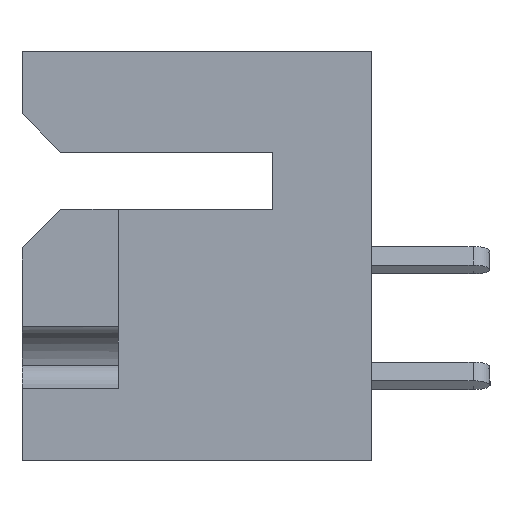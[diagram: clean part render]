
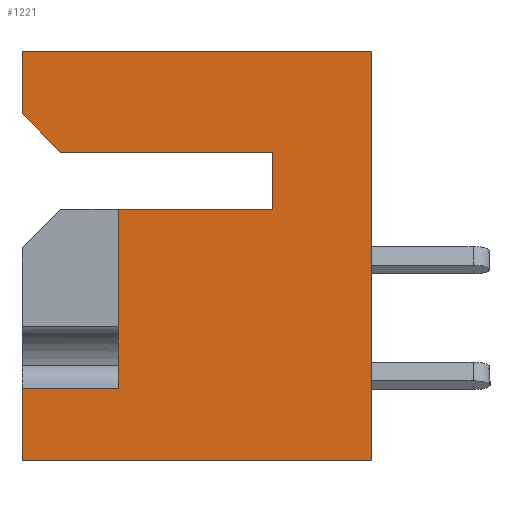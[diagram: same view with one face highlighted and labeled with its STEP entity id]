
A CAD part, left-side view. The second image highlights one B-rep face of the part: STEP entity #1221.
In plain terms, the highlighted planar face has unit normal (-1, 0, 0).
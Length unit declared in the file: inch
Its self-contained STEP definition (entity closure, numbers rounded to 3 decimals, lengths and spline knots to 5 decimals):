
#362 = DIRECTION ( 'NONE',  ( 0., 1., 0. ) ) ;
#945 = VECTOR ( 'NONE', #14442, 39.37008 ) ;
#1119 = ORIENTED_EDGE ( 'NONE', *, *, #4500, .T. ) ;
#1132 = EDGE_CURVE ( 'NONE', #11467, #28084, #12028, .T. ) ;
#1145 = CARTESIAN_POINT ( 'NONE',  ( 0., 0.453, -0.437 ) ) ;
#1221 = ADVANCED_FACE ( 'NONE', ( #16175 ), #7892, .F. ) ;
#1493 = LINE ( 'NONE', #23773, #14653 ) ;
#1674 = AXIS2_PLACEMENT_3D ( 'NONE', #18499, #18599, #3342 ) ;
#2130 = CARTESIAN_POINT ( 'NONE',  ( 0., 0., 0. ) ) ;
#2176 = VECTOR ( 'NONE', #12810, 39.37008 ) ;
#2653 = VECTOR ( 'NONE', #13168, 39.37008 ) ;
#2753 = DIRECTION ( 'NONE',  ( 0., 0., 1. ) ) ;
#3054 = CARTESIAN_POINT ( 'NONE',  ( 0., 0.328, -0.205 ) ) ;
#3342 = DIRECTION ( 'NONE',  ( 0., 0., -1. ) ) ;
#3590 = CARTESIAN_POINT ( 'NONE',  ( 0., 0.453, -0.531 ) ) ;
#3618 = DIRECTION ( 'NONE',  ( 0., 1., 0. ) ) ;
#3740 = EDGE_CURVE ( 'NONE', #21282, #23995, #8416, .T. ) ;
#3867 = LINE ( 'NONE', #22936, #25916 ) ;
#4013 = CARTESIAN_POINT ( 'NONE',  ( 0., 0.128, -0.131 ) ) ;
#4500 = EDGE_CURVE ( 'NONE', #8848, #18688, #3867, .T. ) ;
#4705 = CARTESIAN_POINT ( 'NONE',  ( 0., 0.128, -0.131 ) ) ;
#5362 = VECTOR ( 'NONE', #2753, 39.37008 ) ;
#6960 = EDGE_CURVE ( 'NONE', #21282, #28044, #8560, .T. ) ;
#7069 = CARTESIAN_POINT ( 'NONE',  ( 0., 0.328, -0.437 ) ) ;
#7250 = EDGE_CURVE ( 'NONE', #8031, #23120, #27135, .T. ) ;
#7589 = VECTOR ( 'NONE', #8153, 39.37008 ) ;
#7639 = EDGE_CURVE ( 'NONE', #23120, #28044, #24758, .T. ) ;
#7892 = PLANE ( 'NONE',  #1674 ) ;
#8031 = VERTEX_POINT ( 'NONE', #22704 ) ;
#8153 = DIRECTION ( 'NONE',  ( 0., 0., 1. ) ) ;
#8416 = LINE ( 'NONE', #19460, #2176 ) ;
#8560 = LINE ( 'NONE', #8652, #2653 ) ;
#8652 = CARTESIAN_POINT ( 'NONE',  ( 0., 0.403, -0.131 ) ) ;
#8705 = EDGE_CURVE ( 'NONE', #18688, #21297, #10562, .T. ) ;
#8848 = VERTEX_POINT ( 'NONE', #3590 ) ;
#9035 = VECTOR ( 'NONE', #362, 39.37008 ) ;
#9181 = CARTESIAN_POINT ( 'NONE',  ( 0., 0.328, -0.205 ) ) ;
#9204 = VERTEX_POINT ( 'NONE', #1145 ) ;
#9658 = EDGE_CURVE ( 'NONE', #8848, #9204, #23462, .T. ) ;
#10082 = VECTOR ( 'NONE', #25628, 39.37008 ) ;
#10555 = CARTESIAN_POINT ( 'NONE',  ( 0., 0.453, 0. ) ) ;
#10562 = LINE ( 'NONE', #13758, #5362 ) ;
#11389 = DIRECTION ( 'NONE',  ( 0., 0., 1. ) ) ;
#11467 = VERTEX_POINT ( 'NONE', #19345 ) ;
#12028 = LINE ( 'NONE', #3054, #945 ) ;
#12146 = LINE ( 'NONE', #19001, #10082 ) ;
#12249 = ORIENTED_EDGE ( 'NONE', *, *, #22726, .F. ) ;
#12333 = VECTOR ( 'NONE', #3618, 39.37008 ) ;
#12810 = DIRECTION ( 'NONE',  ( 0., 0., 1. ) ) ;
#12942 = CARTESIAN_POINT ( 'NONE',  ( 0., 0.403, -0.131 ) ) ;
#13168 = DIRECTION ( 'NONE',  ( 0., -0.707, -0.707 ) ) ;
#13758 = CARTESIAN_POINT ( 'NONE',  ( 0., 0., 0. ) ) ;
#13984 = DIRECTION ( 'NONE',  ( 0., -1., 0. ) ) ;
#14442 = DIRECTION ( 'NONE',  ( 0., 0., 1. ) ) ;
#14653 = VECTOR ( 'NONE', #23077, 39.37008 ) ;
#15506 = ORIENTED_EDGE ( 'NONE', *, *, #8705, .T. ) ;
#16032 = ORIENTED_EDGE ( 'NONE', *, *, #9658, .F. ) ;
#16175 = FACE_OUTER_BOUND ( 'NONE', #20472, .T. ) ;
#16934 = ORIENTED_EDGE ( 'NONE', *, *, #20700, .T. ) ;
#18499 = CARTESIAN_POINT ( 'NONE',  ( 0., 0.453, 0. ) ) ;
#18599 = DIRECTION ( 'NONE',  ( 1., 0., 0. ) ) ;
#18688 = VERTEX_POINT ( 'NONE', #24223 ) ;
#19001 = CARTESIAN_POINT ( 'NONE',  ( 0., 0.453, 0. ) ) ;
#19345 = CARTESIAN_POINT ( 'NONE',  ( 0., 0.328, -0.437 ) ) ;
#19408 = CARTESIAN_POINT ( 'NONE',  ( 0., 0.128, -0.131 ) ) ;
#19460 = CARTESIAN_POINT ( 'NONE',  ( 0., 0.453, 0. ) ) ;
#20472 = EDGE_LOOP ( 'NONE', ( #16934, #16032, #1119, #15506, #12249, #21397, #25653, #26553, #27632, #27883, #26038 ) ) ;
#20700 = EDGE_CURVE ( 'NONE', #11467, #9204, #25215, .T. ) ;
#21282 = VERTEX_POINT ( 'NONE', #26244 ) ;
#21297 = VERTEX_POINT ( 'NONE', #2130 ) ;
#21397 = ORIENTED_EDGE ( 'NONE', *, *, #3740, .F. ) ;
#22704 = CARTESIAN_POINT ( 'NONE',  ( 0., 0.128, -0.205 ) ) ;
#22726 = EDGE_CURVE ( 'NONE', #23995, #21297, #12146, .T. ) ;
#22936 = CARTESIAN_POINT ( 'NONE',  ( 0., 0.453, -0.531 ) ) ;
#23077 = DIRECTION ( 'NONE',  ( 0., 1., 0. ) ) ;
#23120 = VERTEX_POINT ( 'NONE', #4705 ) ;
#23462 = LINE ( 'NONE', #26054, #7589 ) ;
#23773 = CARTESIAN_POINT ( 'NONE',  ( 0., 0.128, -0.205 ) ) ;
#23995 = VERTEX_POINT ( 'NONE', #10555 ) ;
#24223 = CARTESIAN_POINT ( 'NONE',  ( 0., 0., -0.531 ) ) ;
#24758 = LINE ( 'NONE', #4013, #12333 ) ;
#25215 = LINE ( 'NONE', #7069, #9035 ) ;
#25628 = DIRECTION ( 'NONE',  ( 0., -1., 0. ) ) ;
#25653 = ORIENTED_EDGE ( 'NONE', *, *, #6960, .T. ) ;
#25916 = VECTOR ( 'NONE', #13984, 39.37008 ) ;
#26038 = ORIENTED_EDGE ( 'NONE', *, *, #1132, .F. ) ;
#26054 = CARTESIAN_POINT ( 'NONE',  ( 0., 0.453, 0. ) ) ;
#26244 = CARTESIAN_POINT ( 'NONE',  ( 0., 0.453, -0.081 ) ) ;
#26466 = VECTOR ( 'NONE', #11389, 39.37008 ) ;
#26553 = ORIENTED_EDGE ( 'NONE', *, *, #7639, .F. ) ;
#27135 = LINE ( 'NONE', #19408, #26466 ) ;
#27205 = EDGE_CURVE ( 'NONE', #8031, #28084, #1493, .T. ) ;
#27632 = ORIENTED_EDGE ( 'NONE', *, *, #7250, .F. ) ;
#27883 = ORIENTED_EDGE ( 'NONE', *, *, #27205, .T. ) ;
#28044 = VERTEX_POINT ( 'NONE', #12942 ) ;
#28084 = VERTEX_POINT ( 'NONE', #9181 ) ;
